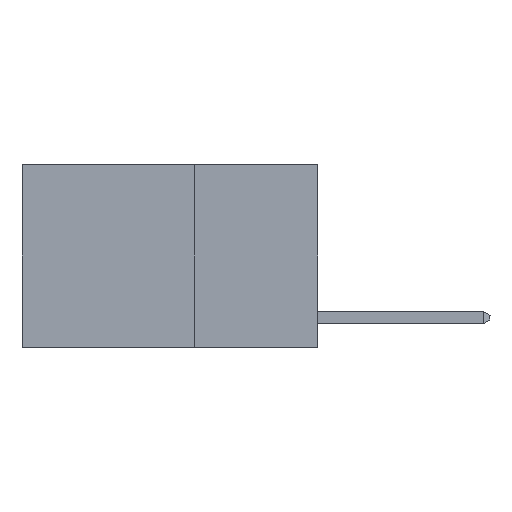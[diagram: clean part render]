
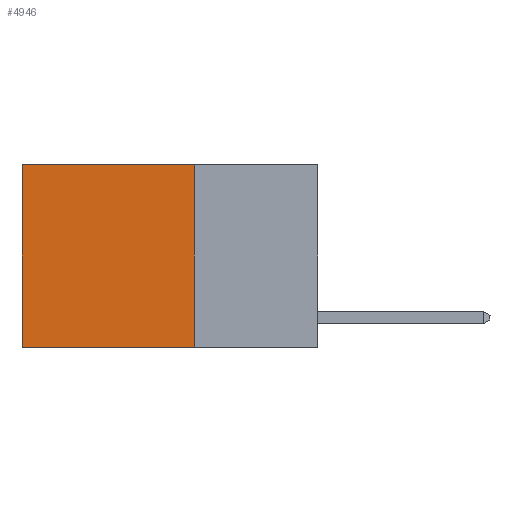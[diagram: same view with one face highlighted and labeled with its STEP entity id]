
A CAD part, left-side view. The second image highlights one B-rep face of the part: STEP entity #4946.
In plain terms, the highlighted planar face has unit normal (-1, 0, 0).
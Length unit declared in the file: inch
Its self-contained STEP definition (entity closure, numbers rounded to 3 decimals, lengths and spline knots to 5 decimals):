
#6 = DIRECTION ( 'NONE',  ( 0., 1., 0. ) ) ;
#68 = CARTESIAN_POINT ( 'NONE',  ( 0.2625, 0.25, 0. ) ) ;
#249 = VERTEX_POINT ( 'NONE', #68 ) ;
#568 = ORIENTED_EDGE ( 'NONE', *, *, #5291, .F. ) ;
#805 = ORIENTED_EDGE ( 'NONE', *, *, #7358, .T. ) ;
#955 = LINE ( 'NONE', #1429, #2765 ) ;
#1233 = DIRECTION ( 'NONE',  ( 0., 0., -1. ) ) ;
#1429 = CARTESIAN_POINT ( 'NONE',  ( 0.2625, 0.25, 0. ) ) ;
#1557 = DIRECTION ( 'NONE',  ( 0., 0., -1. ) ) ;
#1645 = DIRECTION ( 'NONE',  ( 1., 0., 0. ) ) ;
#2436 = EDGE_LOOP ( 'NONE', ( #805, #568, #5335, #4368 ) ) ;
#2719 = CARTESIAN_POINT ( 'NONE',  ( 0.2625, 0.25, -0.37 ) ) ;
#2765 = VECTOR ( 'NONE', #3456, 39.37008 ) ;
#2792 = FACE_OUTER_BOUND ( 'NONE', #2436, .T. ) ;
#3008 = CARTESIAN_POINT ( 'NONE',  ( 0.2625, 0.25, 0. ) ) ;
#3047 = CARTESIAN_POINT ( 'NONE',  ( 0.2625, 0.6, 0. ) ) ;
#3150 = VECTOR ( 'NONE', #7563, 39.37008 ) ;
#3181 = AXIS2_PLACEMENT_3D ( 'NONE', #5551, #1645, #1557 ) ;
#3262 = CARTESIAN_POINT ( 'NONE',  ( 0.2625, 0.6, -0.37 ) ) ;
#3304 = VECTOR ( 'NONE', #1233, 39.37008 ) ;
#3329 = CARTESIAN_POINT ( 'NONE',  ( 0.2625, 0.25, -0.37 ) ) ;
#3456 = DIRECTION ( 'NONE',  ( 0., 1., 0. ) ) ;
#3664 = LINE ( 'NONE', #3008, #3150 ) ;
#3743 = LINE ( 'NONE', #3047, #3304 ) ;
#4023 = EDGE_CURVE ( 'NONE', #249, #5332, #3664, .T. ) ;
#4368 = ORIENTED_EDGE ( 'NONE', *, *, #4869, .T. ) ;
#4869 = EDGE_CURVE ( 'NONE', #249, #7838, #955, .T. ) ;
#4946 = ADVANCED_FACE ( 'NONE', ( #2792 ), #7449, .F. ) ;
#5291 = EDGE_CURVE ( 'NONE', #5332, #7497, #5375, .T. ) ;
#5332 = VERTEX_POINT ( 'NONE', #3329 ) ;
#5335 = ORIENTED_EDGE ( 'NONE', *, *, #4023, .F. ) ;
#5375 = LINE ( 'NONE', #2719, #8058 ) ;
#5551 = CARTESIAN_POINT ( 'NONE',  ( 0.2625, 0.25, 0. ) ) ;
#5698 = CARTESIAN_POINT ( 'NONE',  ( 0.2625, 0.6, 0. ) ) ;
#7358 = EDGE_CURVE ( 'NONE', #7838, #7497, #3743, .T. ) ;
#7449 = PLANE ( 'NONE',  #3181 ) ;
#7497 = VERTEX_POINT ( 'NONE', #3262 ) ;
#7563 = DIRECTION ( 'NONE',  ( 0., 0., -1. ) ) ;
#7838 = VERTEX_POINT ( 'NONE', #5698 ) ;
#8058 = VECTOR ( 'NONE', #6, 39.37008 ) ;
